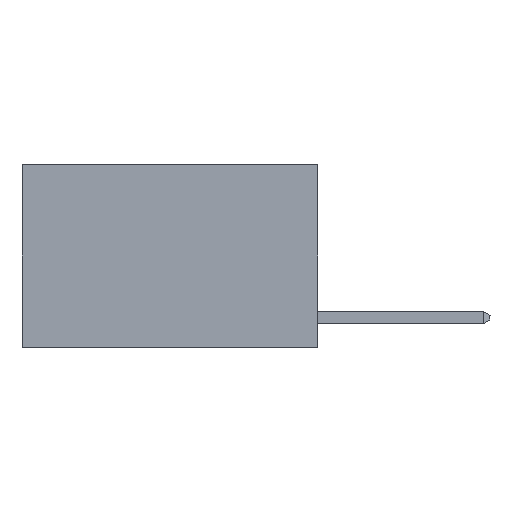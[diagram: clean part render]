
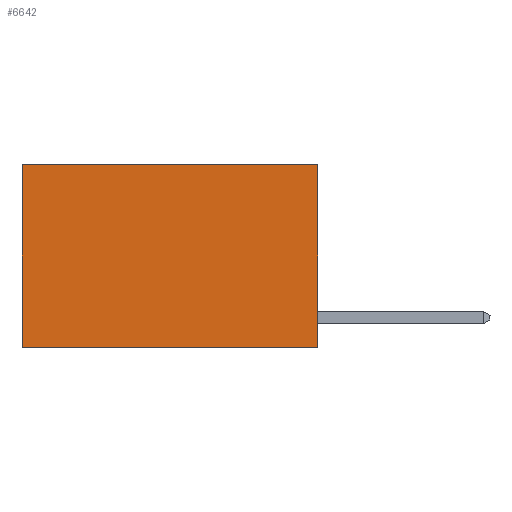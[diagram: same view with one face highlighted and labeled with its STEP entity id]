
A CAD part, left-side view. The second image highlights one B-rep face of the part: STEP entity #6642.
In plain terms, the highlighted planar face has unit normal (-1, 0, 0).
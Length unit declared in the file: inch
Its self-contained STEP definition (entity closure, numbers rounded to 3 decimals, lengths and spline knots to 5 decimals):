
#166 = DIRECTION ( 'NONE',  ( 0., 0., -1. ) ) ;
#306 = VERTEX_POINT ( 'NONE', #5740 ) ;
#506 = FACE_OUTER_BOUND ( 'NONE', #2728, .T. ) ;
#952 = ORIENTED_EDGE ( 'NONE', *, *, #5697, .T. ) ;
#1471 = VECTOR ( 'NONE', #7755, 39.37008 ) ;
#1524 = LINE ( 'NONE', #7833, #1471 ) ;
#1756 = EDGE_CURVE ( 'NONE', #6011, #2764, #6859, .T. ) ;
#1841 = DIRECTION ( 'NONE',  ( 0., 0., -1. ) ) ;
#2414 = CARTESIAN_POINT ( 'NONE',  ( 0.2625, 0., -0.37 ) ) ;
#2728 = EDGE_LOOP ( 'NONE', ( #4944, #4331, #5675, #952 ) ) ;
#2764 = VERTEX_POINT ( 'NONE', #6075 ) ;
#2957 = AXIS2_PLACEMENT_3D ( 'NONE', #4501, #4402, #4383 ) ;
#2984 = DIRECTION ( 'NONE',  ( 0., 1., 0. ) ) ;
#3023 = CARTESIAN_POINT ( 'NONE',  ( 0.2625, 0., 0. ) ) ;
#3407 = EDGE_CURVE ( 'NONE', #2764, #6008, #5680, .T. ) ;
#4331 = ORIENTED_EDGE ( 'NONE', *, *, #3407, .F. ) ;
#4383 = DIRECTION ( 'NONE',  ( 0., 0., -1. ) ) ;
#4402 = DIRECTION ( 'NONE',  ( 1., 0., 0. ) ) ;
#4469 = PLANE ( 'NONE',  #2957 ) ;
#4501 = CARTESIAN_POINT ( 'NONE',  ( 0.2625, 0., 0. ) ) ;
#4944 = ORIENTED_EDGE ( 'NONE', *, *, #7423, .T. ) ;
#5599 = VECTOR ( 'NONE', #2984, 39.37008 ) ;
#5675 = ORIENTED_EDGE ( 'NONE', *, *, #1756, .F. ) ;
#5680 = LINE ( 'NONE', #2414, #5599 ) ;
#5697 = EDGE_CURVE ( 'NONE', #6011, #306, #1524, .T. ) ;
#5740 = CARTESIAN_POINT ( 'NONE',  ( 0.2625, 0.6, 0. ) ) ;
#5782 = LINE ( 'NONE', #6722, #7339 ) ;
#6008 = VERTEX_POINT ( 'NONE', #6976 ) ;
#6011 = VERTEX_POINT ( 'NONE', #6961 ) ;
#6075 = CARTESIAN_POINT ( 'NONE',  ( 0.2625, 0., -0.37 ) ) ;
#6642 = ADVANCED_FACE ( 'NONE', ( #506 ), #4469, .F. ) ;
#6696 = VECTOR ( 'NONE', #166, 39.37008 ) ;
#6722 = CARTESIAN_POINT ( 'NONE',  ( 0.2625, 0.6, 0. ) ) ;
#6859 = LINE ( 'NONE', #3023, #6696 ) ;
#6961 = CARTESIAN_POINT ( 'NONE',  ( 0.2625, 0., 0. ) ) ;
#6976 = CARTESIAN_POINT ( 'NONE',  ( 0.2625, 0.6, -0.37 ) ) ;
#7339 = VECTOR ( 'NONE', #1841, 39.37008 ) ;
#7423 = EDGE_CURVE ( 'NONE', #306, #6008, #5782, .T. ) ;
#7755 = DIRECTION ( 'NONE',  ( 0., 1., 0. ) ) ;
#7833 = CARTESIAN_POINT ( 'NONE',  ( 0.2625, 0., 0. ) ) ;
